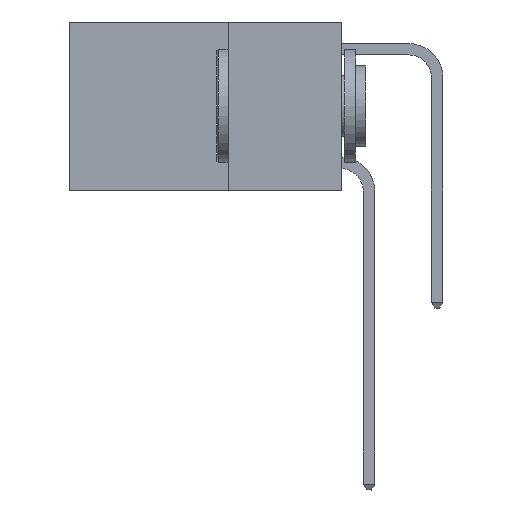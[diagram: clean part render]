
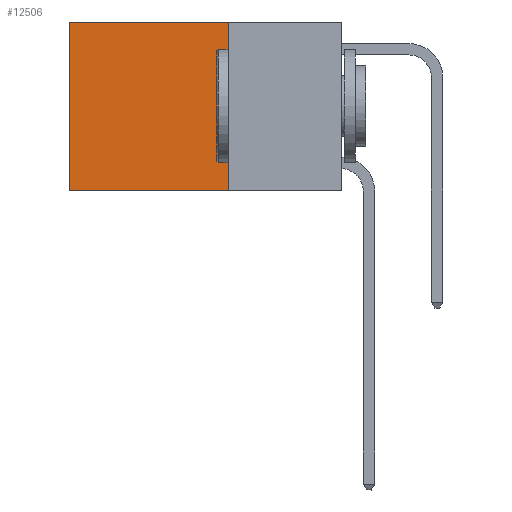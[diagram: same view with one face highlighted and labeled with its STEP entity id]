
A CAD part, left-side view. The second image highlights one B-rep face of the part: STEP entity #12506.
In plain terms, the highlighted planar face has unit normal (-1, 0, 0).
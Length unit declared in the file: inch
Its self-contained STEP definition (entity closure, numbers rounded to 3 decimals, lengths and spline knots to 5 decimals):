
#6 = VECTOR ( 'NONE', #17126, 39.37008 ) ;
#100 = VERTEX_POINT ( 'NONE', #437 ) ;
#414 = ORIENTED_EDGE ( 'NONE', *, *, #11663, .T. ) ;
#437 = CARTESIAN_POINT ( 'NONE',  ( 0.2625, 0.25, -0.37 ) ) ;
#767 = FACE_OUTER_BOUND ( 'NONE', #10367, .T. ) ;
#2256 = VECTOR ( 'NONE', #24545, 39.37008 ) ;
#2332 = DIRECTION ( 'NONE',  ( 0., 1., 0. ) ) ;
#3742 = CARTESIAN_POINT ( 'NONE',  ( 0.2625, 0.6, -0.37 ) ) ;
#3895 = LINE ( 'NONE', #19698, #2256 ) ;
#4131 = LINE ( 'NONE', #20844, #23933 ) ;
#5030 = CARTESIAN_POINT ( 'NONE',  ( 0.2625, 0.25, -0.37 ) ) ;
#5206 = DIRECTION ( 'NONE',  ( 0., 1., 0. ) ) ;
#5935 = DIRECTION ( 'NONE',  ( 0., 0., -1. ) ) ;
#6985 = CARTESIAN_POINT ( 'NONE',  ( 0.2625, 0.25, 0. ) ) ;
#10112 = LINE ( 'NONE', #32532, #6 ) ;
#10306 = ORIENTED_EDGE ( 'NONE', *, *, #17236, .T. ) ;
#10367 = EDGE_LOOP ( 'NONE', ( #414, #20929, #11216, #10306 ) ) ;
#10517 = VERTEX_POINT ( 'NONE', #3742 ) ;
#11216 = ORIENTED_EDGE ( 'NONE', *, *, #28679, .F. ) ;
#11663 = EDGE_CURVE ( 'NONE', #18421, #10517, #3895, .T. ) ;
#12506 = ADVANCED_FACE ( 'NONE', ( #767 ), #21570, .F. ) ;
#17126 = DIRECTION ( 'NONE',  ( 0., 0., -1. ) ) ;
#17236 = EDGE_CURVE ( 'NONE', #17696, #18421, #4131, .T. ) ;
#17696 = VERTEX_POINT ( 'NONE', #6985 ) ;
#18421 = VERTEX_POINT ( 'NONE', #21166 ) ;
#18561 = AXIS2_PLACEMENT_3D ( 'NONE', #31336, #19152, #5935 ) ;
#19152 = DIRECTION ( 'NONE',  ( 1., 0., 0. ) ) ;
#19698 = CARTESIAN_POINT ( 'NONE',  ( 0.2625, 0.6, 0. ) ) ;
#20844 = CARTESIAN_POINT ( 'NONE',  ( 0.2625, 0.25, 0. ) ) ;
#20929 = ORIENTED_EDGE ( 'NONE', *, *, #30972, .F. ) ;
#21166 = CARTESIAN_POINT ( 'NONE',  ( 0.2625, 0.6, 0. ) ) ;
#21570 = PLANE ( 'NONE',  #18561 ) ;
#23330 = LINE ( 'NONE', #5030, #31427 ) ;
#23933 = VECTOR ( 'NONE', #5206, 39.37008 ) ;
#24545 = DIRECTION ( 'NONE',  ( 0., 0., -1. ) ) ;
#28679 = EDGE_CURVE ( 'NONE', #17696, #100, #10112, .T. ) ;
#30972 = EDGE_CURVE ( 'NONE', #100, #10517, #23330, .T. ) ;
#31336 = CARTESIAN_POINT ( 'NONE',  ( 0.2625, 0.25, 0. ) ) ;
#31427 = VECTOR ( 'NONE', #2332, 39.37008 ) ;
#32532 = CARTESIAN_POINT ( 'NONE',  ( 0.2625, 0.25, 0. ) ) ;
